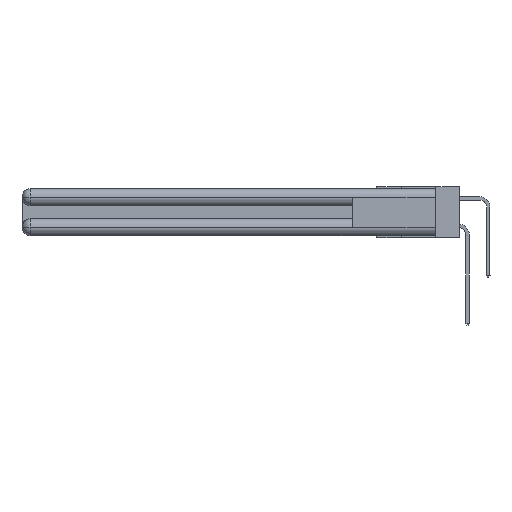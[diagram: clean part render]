
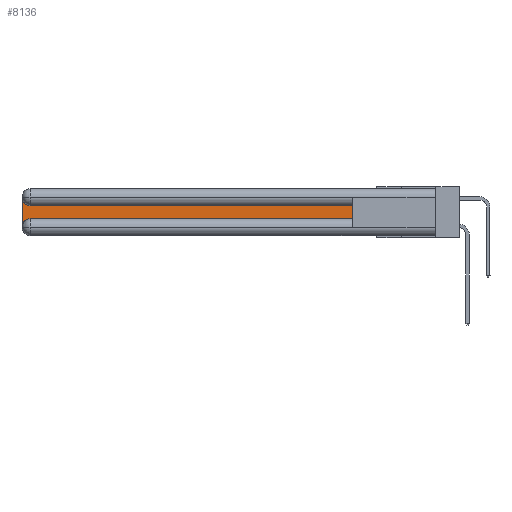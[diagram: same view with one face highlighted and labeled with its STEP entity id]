
A CAD part, left-side view. The second image highlights one B-rep face of the part: STEP entity #8136.
In plain terms, the highlighted planar face has unit normal (-1, 0, 0).
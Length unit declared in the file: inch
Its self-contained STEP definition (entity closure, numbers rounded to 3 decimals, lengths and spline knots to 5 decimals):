
#514 = CARTESIAN_POINT ( 'NONE',  ( 0.075, 0.6, -0.1225 ) ) ;
#579 = VERTEX_POINT ( 'NONE', #16151 ) ;
#804 = ORIENTED_EDGE ( 'NONE', *, *, #4539, .T. ) ;
#811 = CARTESIAN_POINT ( 'NONE',  ( 0.075, 3., -0.1225 ) ) ;
#1259 = DIRECTION ( 'NONE',  ( 0., -1., 0. ) ) ;
#1301 = VERTEX_POINT ( 'NONE', #3298 ) ;
#1333 = FACE_OUTER_BOUND ( 'NONE', #15633, .T. ) ;
#1555 = LINE ( 'NONE', #26266, #24020 ) ;
#2470 = EDGE_CURVE ( 'NONE', #14223, #1301, #19363, .T. ) ;
#3298 = CARTESIAN_POINT ( 'NONE',  ( 0.075, 3., -0.0625 ) ) ;
#3883 = LINE ( 'NONE', #514, #8309 ) ;
#4539 = EDGE_CURVE ( 'NONE', #14056, #24303, #7970, .T. ) ;
#5302 = CARTESIAN_POINT ( 'NONE',  ( 0.075, 3., -0.2775 ) ) ;
#5427 = DIRECTION ( 'NONE',  ( 0., 0., -1. ) ) ;
#5670 = ORIENTED_EDGE ( 'NONE', *, *, #2470, .T. ) ;
#5898 = ORIENTED_EDGE ( 'NONE', *, *, #23734, .T. ) ;
#6321 = PLANE ( 'NONE',  #26264 ) ;
#7111 = DIRECTION ( 'NONE',  ( 1., 0., 0. ) ) ;
#7970 = LINE ( 'NONE', #21559, #11184 ) ;
#8136 = ADVANCED_FACE ( 'NONE', ( #1333 ), #6321, .F. ) ;
#8309 = VECTOR ( 'NONE', #15584, 39.37008 ) ;
#9957 = CARTESIAN_POINT ( 'NONE',  ( 0.075, 0.6, -0.1225 ) ) ;
#10073 = CARTESIAN_POINT ( 'NONE',  ( 0.075, 2.94, -0.1225 ) ) ;
#11184 = VECTOR ( 'NONE', #28990, 39.37008 ) ;
#11476 = DIRECTION ( 'NONE',  ( 1., 0., 0. ) ) ;
#12283 = CARTESIAN_POINT ( 'NONE',  ( 0.075, 2.94, -0.2775 ) ) ;
#13248 = DIRECTION ( 'NONE',  ( 1., 0., 0. ) ) ;
#14056 = VERTEX_POINT ( 'NONE', #15377 ) ;
#14223 = VERTEX_POINT ( 'NONE', #10073 ) ;
#15377 = CARTESIAN_POINT ( 'NONE',  ( 0.075, 0.6, -0.2175 ) ) ;
#15552 = ORIENTED_EDGE ( 'NONE', *, *, #31003, .T. ) ;
#15584 = DIRECTION ( 'NONE',  ( 0., 1., 0. ) ) ;
#15633 = EDGE_LOOP ( 'NONE', ( #5898, #5670, #30525, #15552, #19886, #804 ) ) ;
#16151 = CARTESIAN_POINT ( 'NONE',  ( 0.075, 2.94, -0.2175 ) ) ;
#17180 = LINE ( 'NONE', #29299, #25210 ) ;
#18508 = DIRECTION ( 'NONE',  ( 0., 0., -1. ) ) ;
#19363 = CIRCLE ( 'NONE', #30266, 0.06 ) ;
#19886 = ORIENTED_EDGE ( 'NONE', *, *, #29524, .T. ) ;
#21190 = VERTEX_POINT ( 'NONE', #5302 ) ;
#21559 = CARTESIAN_POINT ( 'NONE',  ( 0.075, 0.6, -0.2175 ) ) ;
#23734 = EDGE_CURVE ( 'NONE', #24303, #14223, #3883, .T. ) ;
#24020 = VECTOR ( 'NONE', #5427, 39.37008 ) ;
#24303 = VERTEX_POINT ( 'NONE', #9957 ) ;
#25210 = VECTOR ( 'NONE', #1259, 39.37008 ) ;
#26264 = AXIS2_PLACEMENT_3D ( 'NONE', #811, #11476, #26610 ) ;
#26266 = CARTESIAN_POINT ( 'NONE',  ( 0.075, 3., -0.2175 ) ) ;
#26543 = AXIS2_PLACEMENT_3D ( 'NONE', #12283, #7111, #32691 ) ;
#26610 = DIRECTION ( 'NONE',  ( 0., 0., -1. ) ) ;
#28990 = DIRECTION ( 'NONE',  ( 0., 0., 1. ) ) ;
#29299 = CARTESIAN_POINT ( 'NONE',  ( 0.075, 0.6, -0.2175 ) ) ;
#29326 = CIRCLE ( 'NONE', #26543, 0.06 ) ;
#29524 = EDGE_CURVE ( 'NONE', #579, #14056, #17180, .T. ) ;
#30266 = AXIS2_PLACEMENT_3D ( 'NONE', #31299, #13248, #18508 ) ;
#30525 = ORIENTED_EDGE ( 'NONE', *, *, #32580, .T. ) ;
#31003 = EDGE_CURVE ( 'NONE', #21190, #579, #29326, .T. ) ;
#31299 = CARTESIAN_POINT ( 'NONE',  ( 0.075, 2.94, -0.0625 ) ) ;
#32580 = EDGE_CURVE ( 'NONE', #1301, #21190, #1555, .T. ) ;
#32691 = DIRECTION ( 'NONE',  ( 0., 0., -1. ) ) ;
